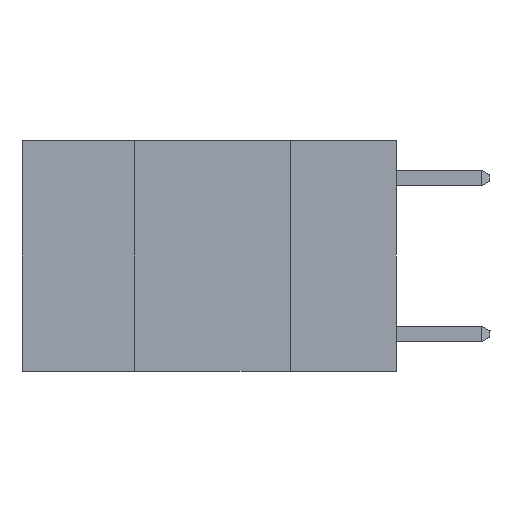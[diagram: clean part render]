
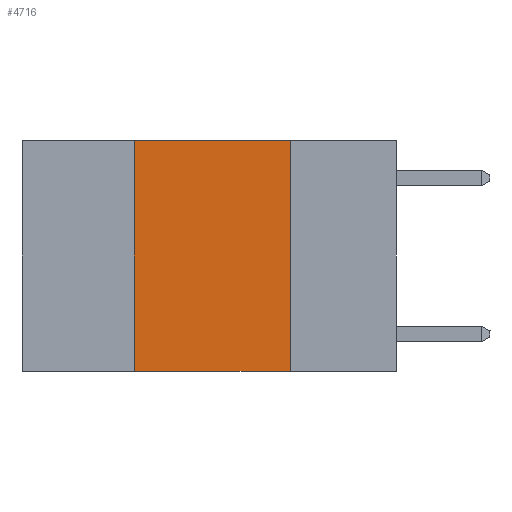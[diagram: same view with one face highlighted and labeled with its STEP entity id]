
A CAD part, left-side view. The second image highlights one B-rep face of the part: STEP entity #4716.
In plain terms, the highlighted planar face has unit normal (-1, 0, 0).
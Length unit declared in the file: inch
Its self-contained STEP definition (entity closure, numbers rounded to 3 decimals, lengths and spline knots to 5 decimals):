
#302 = ORIENTED_EDGE ( 'NONE', *, *, #8015, .F. ) ;
#320 = VERTEX_POINT ( 'NONE', #3550 ) ;
#893 = CARTESIAN_POINT ( 'NONE',  ( 0., 0.17, 0. ) ) ;
#1490 = DIRECTION ( 'NONE',  ( 0., 0., -1. ) ) ;
#1512 = DIRECTION ( 'NONE',  ( 1., 0., 0. ) ) ;
#1566 = PLANE ( 'NONE',  #6740 ) ;
#1632 = CARTESIAN_POINT ( 'NONE',  ( 0., 0.6, 0. ) ) ;
#1788 = LINE ( 'NONE', #7081, #7702 ) ;
#1933 = CARTESIAN_POINT ( 'NONE',  ( 0., 0.6, 0. ) ) ;
#2368 = CARTESIAN_POINT ( 'NONE',  ( 0., 0.42, 0. ) ) ;
#2448 = EDGE_CURVE ( 'NONE', #320, #7118, #1788, .T. ) ;
#2632 = DIRECTION ( 'NONE',  ( 0., 0., 1. ) ) ;
#2771 = LINE ( 'NONE', #2368, #8408 ) ;
#3550 = CARTESIAN_POINT ( 'NONE',  ( 0., 0.42, -0.37 ) ) ;
#3658 = ORIENTED_EDGE ( 'NONE', *, *, #2448, .T. ) ;
#4526 = ORIENTED_EDGE ( 'NONE', *, *, #8900, .F. ) ;
#4616 = VECTOR ( 'NONE', #4780, 39.37008 ) ;
#4716 = ADVANCED_FACE ( 'NONE', ( #8794 ), #1566, .F. ) ;
#4754 = DIRECTION ( 'NONE',  ( 0., 0., -1. ) ) ;
#4780 = DIRECTION ( 'NONE',  ( 0., -1., 0. ) ) ;
#5334 = EDGE_CURVE ( 'NONE', #320, #9413, #2771, .T. ) ;
#6691 = CARTESIAN_POINT ( 'NONE',  ( 0., 0.17, 0. ) ) ;
#6696 = LINE ( 'NONE', #1632, #4616 ) ;
#6740 = AXIS2_PLACEMENT_3D ( 'NONE', #1933, #1512, #1490 ) ;
#6776 = CARTESIAN_POINT ( 'NONE',  ( 0., 0.42, 0. ) ) ;
#7081 = CARTESIAN_POINT ( 'NONE',  ( 0., 0.6, -0.37 ) ) ;
#7111 = ORIENTED_EDGE ( 'NONE', *, *, #5334, .F. ) ;
#7118 = VERTEX_POINT ( 'NONE', #8419 ) ;
#7148 = EDGE_LOOP ( 'NONE', ( #302, #4526, #7111, #3658 ) ) ;
#7284 = VECTOR ( 'NONE', #4754, 39.37008 ) ;
#7702 = VECTOR ( 'NONE', #8471, 39.37008 ) ;
#8015 = EDGE_CURVE ( 'NONE', #8414, #7118, #9189, .T. ) ;
#8408 = VECTOR ( 'NONE', #2632, 39.37008 ) ;
#8414 = VERTEX_POINT ( 'NONE', #6691 ) ;
#8419 = CARTESIAN_POINT ( 'NONE',  ( 0., 0.17, -0.37 ) ) ;
#8471 = DIRECTION ( 'NONE',  ( 0., -1., 0. ) ) ;
#8794 = FACE_OUTER_BOUND ( 'NONE', #7148, .T. ) ;
#8900 = EDGE_CURVE ( 'NONE', #9413, #8414, #6696, .T. ) ;
#9189 = LINE ( 'NONE', #893, #7284 ) ;
#9413 = VERTEX_POINT ( 'NONE', #6776 ) ;
